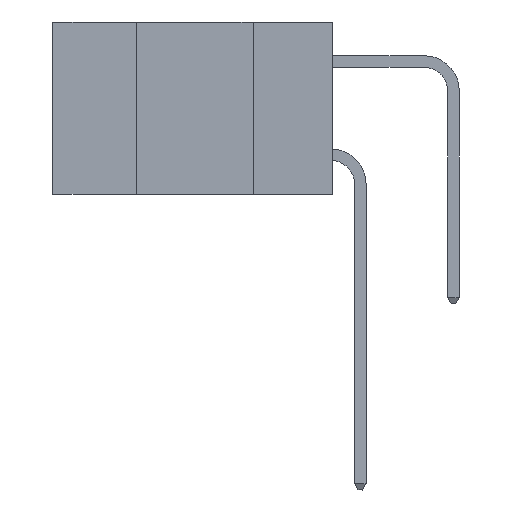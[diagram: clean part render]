
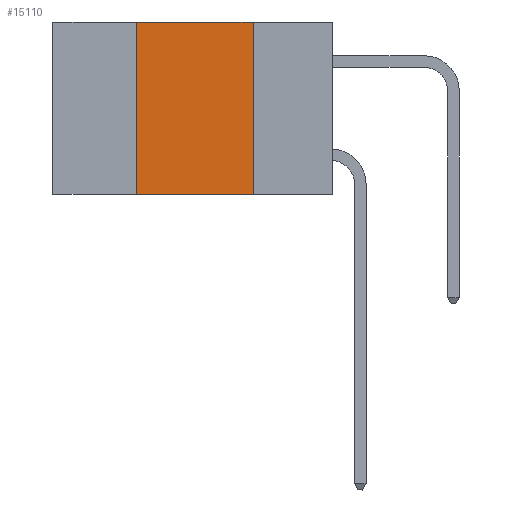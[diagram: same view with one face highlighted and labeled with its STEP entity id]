
A CAD part, left-side view. The second image highlights one B-rep face of the part: STEP entity #15110.
In plain terms, the highlighted planar face has unit normal (-1, 0, 0).
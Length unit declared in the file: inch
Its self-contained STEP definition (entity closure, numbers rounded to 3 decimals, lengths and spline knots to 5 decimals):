
#93 = ORIENTED_EDGE ( 'NONE', *, *, #15859, .F. ) ;
#161 = DIRECTION ( 'NONE',  ( 0., 0., -1. ) ) ;
#713 = CARTESIAN_POINT ( 'NONE',  ( 0., 0.42, -0.37 ) ) ;
#720 = CARTESIAN_POINT ( 'NONE',  ( 0., 0.42, 0. ) ) ;
#970 = FACE_OUTER_BOUND ( 'NONE', #10480, .T. ) ;
#987 = LINE ( 'NONE', #720, #16927 ) ;
#2002 = DIRECTION ( 'NONE',  ( 0., -1., 0. ) ) ;
#2123 = CARTESIAN_POINT ( 'NONE',  ( 0., 0.17, -0.37 ) ) ;
#2836 = PLANE ( 'NONE',  #7568 ) ;
#4354 = LINE ( 'NONE', #24862, #11780 ) ;
#4554 = CARTESIAN_POINT ( 'NONE',  ( 0., 0.17, 0. ) ) ;
#6158 = CARTESIAN_POINT ( 'NONE',  ( 0., 0.6, 0. ) ) ;
#7568 = AXIS2_PLACEMENT_3D ( 'NONE', #24753, #16202, #22891 ) ;
#10123 = ORIENTED_EDGE ( 'NONE', *, *, #18783, .F. ) ;
#10244 = VERTEX_POINT ( 'NONE', #2123 ) ;
#10311 = VECTOR ( 'NONE', #161, 39.37008 ) ;
#10480 = EDGE_LOOP ( 'NONE', ( #25097, #93, #10123, #25200 ) ) ;
#11780 = VECTOR ( 'NONE', #11815, 39.37008 ) ;
#11815 = DIRECTION ( 'NONE',  ( 0., -1., 0. ) ) ;
#13147 = CARTESIAN_POINT ( 'NONE',  ( 0., 0.17, 0. ) ) ;
#15110 = ADVANCED_FACE ( 'NONE', ( #970 ), #2836, .F. ) ;
#15859 = EDGE_CURVE ( 'NONE', #27422, #19020, #17903, .T. ) ;
#16202 = DIRECTION ( 'NONE',  ( 1., 0., 0. ) ) ;
#16927 = VECTOR ( 'NONE', #17881, 39.37008 ) ;
#17166 = EDGE_CURVE ( 'NONE', #19020, #10244, #17485, .T. ) ;
#17485 = LINE ( 'NONE', #13147, #10311 ) ;
#17881 = DIRECTION ( 'NONE',  ( 0., 0., 1. ) ) ;
#17903 = LINE ( 'NONE', #6158, #25035 ) ;
#18783 = EDGE_CURVE ( 'NONE', #20910, #27422, #987, .T. ) ;
#19020 = VERTEX_POINT ( 'NONE', #4554 ) ;
#19139 = EDGE_CURVE ( 'NONE', #20910, #10244, #4354, .T. ) ;
#20910 = VERTEX_POINT ( 'NONE', #713 ) ;
#22891 = DIRECTION ( 'NONE',  ( 0., 0., -1. ) ) ;
#23784 = CARTESIAN_POINT ( 'NONE',  ( 0., 0.42, 0. ) ) ;
#24753 = CARTESIAN_POINT ( 'NONE',  ( 0., 0.6, 0. ) ) ;
#24862 = CARTESIAN_POINT ( 'NONE',  ( 0., 0.6, -0.37 ) ) ;
#25035 = VECTOR ( 'NONE', #2002, 39.37008 ) ;
#25097 = ORIENTED_EDGE ( 'NONE', *, *, #17166, .F. ) ;
#25200 = ORIENTED_EDGE ( 'NONE', *, *, #19139, .T. ) ;
#27422 = VERTEX_POINT ( 'NONE', #23784 ) ;
